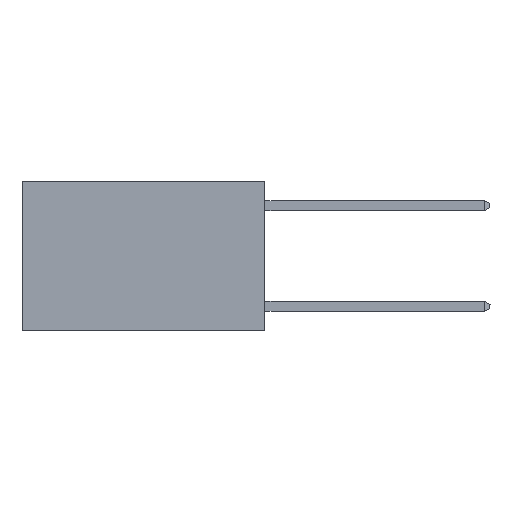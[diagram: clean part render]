
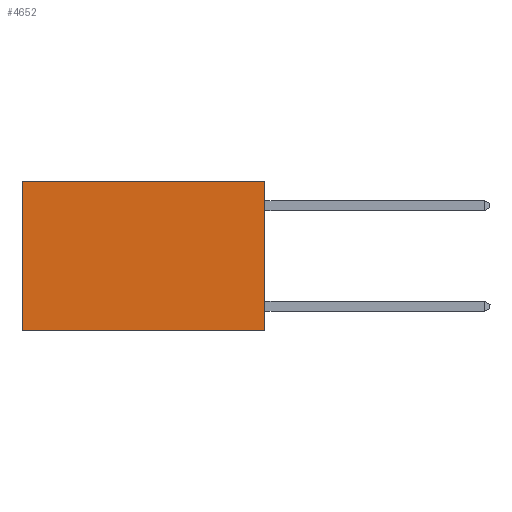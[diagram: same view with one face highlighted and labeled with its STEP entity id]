
A CAD part, left-side view. The second image highlights one B-rep face of the part: STEP entity #4652.
In plain terms, the highlighted planar face has unit normal (-1, 0, 0).
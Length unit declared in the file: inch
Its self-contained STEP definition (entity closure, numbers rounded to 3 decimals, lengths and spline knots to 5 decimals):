
#112 = VECTOR ( 'NONE', #9848, 39.37008 ) ;
#242 = DIRECTION ( 'NONE',  ( 0., 1., 0. ) ) ;
#419 = ORIENTED_EDGE ( 'NONE', *, *, #7252, .F. ) ;
#1086 = LINE ( 'NONE', #10672, #10095 ) ;
#2008 = CARTESIAN_POINT ( 'NONE',  ( 0.2625, 0., 0. ) ) ;
#2284 = ORIENTED_EDGE ( 'NONE', *, *, #15685, .T. ) ;
#2709 = FACE_OUTER_BOUND ( 'NONE', #4123, .T. ) ;
#2783 = ORIENTED_EDGE ( 'NONE', *, *, #12454, .T. ) ;
#3890 = DIRECTION ( 'NONE',  ( 0., 0., -1. ) ) ;
#4104 = VECTOR ( 'NONE', #242, 39.37008 ) ;
#4123 = EDGE_LOOP ( 'NONE', ( #2284, #419, #5675, #2783 ) ) ;
#4497 = VERTEX_POINT ( 'NONE', #14459 ) ;
#4652 = ADVANCED_FACE ( 'NONE', ( #2709 ), #9941, .F. ) ;
#5031 = CARTESIAN_POINT ( 'NONE',  ( 0.2625, 0., 0. ) ) ;
#5183 = CARTESIAN_POINT ( 'NONE',  ( 0.2625, 0., -0.37 ) ) ;
#5675 = ORIENTED_EDGE ( 'NONE', *, *, #9459, .F. ) ;
#5920 = DIRECTION ( 'NONE',  ( 0., 0., -1. ) ) ;
#7252 = EDGE_CURVE ( 'NONE', #8512, #4497, #10915, .T. ) ;
#8512 = VERTEX_POINT ( 'NONE', #5183 ) ;
#8667 = CARTESIAN_POINT ( 'NONE',  ( 0.2625, 0.6, 0. ) ) ;
#9350 = DIRECTION ( 'NONE',  ( 0., 1., 0. ) ) ;
#9459 = EDGE_CURVE ( 'NONE', #11379, #8512, #1086, .T. ) ;
#9848 = DIRECTION ( 'NONE',  ( 0., 0., -1. ) ) ;
#9941 = PLANE ( 'NONE',  #15089 ) ;
#10095 = VECTOR ( 'NONE', #5920, 39.37008 ) ;
#10672 = CARTESIAN_POINT ( 'NONE',  ( 0.2625, 0., 0. ) ) ;
#10915 = LINE ( 'NONE', #14836, #4104 ) ;
#11135 = DIRECTION ( 'NONE',  ( 1., 0., 0. ) ) ;
#11379 = VERTEX_POINT ( 'NONE', #5031 ) ;
#11990 = CARTESIAN_POINT ( 'NONE',  ( 0.2625, 0.6, 0. ) ) ;
#12085 = VECTOR ( 'NONE', #9350, 39.37008 ) ;
#12454 = EDGE_CURVE ( 'NONE', #11379, #13715, #13216, .T. ) ;
#13216 = LINE ( 'NONE', #2008, #12085 ) ;
#13509 = LINE ( 'NONE', #8667, #112 ) ;
#13715 = VERTEX_POINT ( 'NONE', #11990 ) ;
#14459 = CARTESIAN_POINT ( 'NONE',  ( 0.2625, 0.6, -0.37 ) ) ;
#14665 = CARTESIAN_POINT ( 'NONE',  ( 0.2625, 0., 0. ) ) ;
#14836 = CARTESIAN_POINT ( 'NONE',  ( 0.2625, 0., -0.37 ) ) ;
#15089 = AXIS2_PLACEMENT_3D ( 'NONE', #14665, #11135, #3890 ) ;
#15685 = EDGE_CURVE ( 'NONE', #13715, #4497, #13509, .T. ) ;
